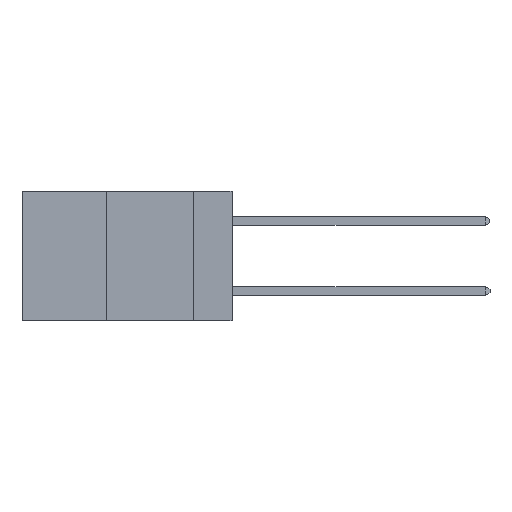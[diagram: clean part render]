
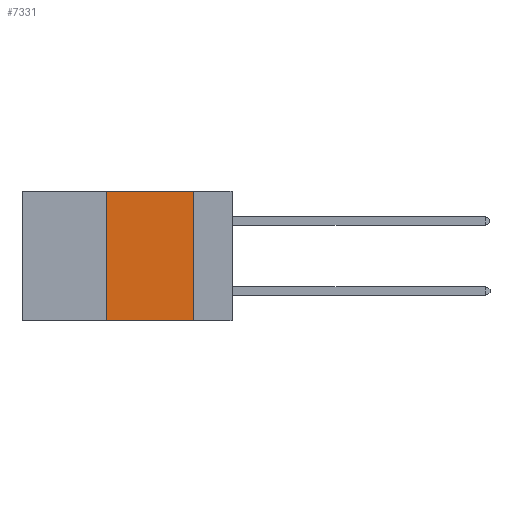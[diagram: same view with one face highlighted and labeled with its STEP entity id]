
A CAD part, left-side view. The second image highlights one B-rep face of the part: STEP entity #7331.
In plain terms, the highlighted planar face has unit normal (-1, 0, 0).
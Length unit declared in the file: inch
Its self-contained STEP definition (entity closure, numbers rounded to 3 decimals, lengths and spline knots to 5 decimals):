
#39 = LINE ( 'NONE', #3463, #8463 ) ;
#714 = ORIENTED_EDGE ( 'NONE', *, *, #12459, .F. ) ;
#884 = DIRECTION ( 'NONE',  ( 0., -1., 0. ) ) ;
#1020 = FACE_OUTER_BOUND ( 'NONE', #5748, .T. ) ;
#1341 = CARTESIAN_POINT ( 'NONE',  ( 0., 0.36, -0.37 ) ) ;
#2169 = VERTEX_POINT ( 'NONE', #8030 ) ;
#2723 = CARTESIAN_POINT ( 'NONE',  ( 0., 0.6, 0. ) ) ;
#2882 = VECTOR ( 'NONE', #884, 39.37008 ) ;
#3002 = EDGE_CURVE ( 'NONE', #5254, #2169, #13405, .T. ) ;
#3463 = CARTESIAN_POINT ( 'NONE',  ( 0., 0.36, 0. ) ) ;
#3580 = CARTESIAN_POINT ( 'NONE',  ( 0., 0.11, 0. ) ) ;
#3927 = VECTOR ( 'NONE', #16142, 39.37008 ) ;
#5190 = EDGE_CURVE ( 'NONE', #8647, #16132, #12346, .T. ) ;
#5254 = VERTEX_POINT ( 'NONE', #1341 ) ;
#5429 = PLANE ( 'NONE',  #18193 ) ;
#5748 = EDGE_LOOP ( 'NONE', ( #714, #13104, #17016, #14029 ) ) ;
#6553 = DIRECTION ( 'NONE',  ( 0., 0., -1. ) ) ;
#7331 = ADVANCED_FACE ( 'NONE', ( #1020 ), #5429, .F. ) ;
#8030 = CARTESIAN_POINT ( 'NONE',  ( 0., 0.11, -0.37 ) ) ;
#8449 = DIRECTION ( 'NONE',  ( 0., 0., -1. ) ) ;
#8463 = VECTOR ( 'NONE', #12419, 39.37008 ) ;
#8647 = VERTEX_POINT ( 'NONE', #14761 ) ;
#9821 = CARTESIAN_POINT ( 'NONE',  ( 0., 0.6, -0.37 ) ) ;
#12346 = LINE ( 'NONE', #2723, #3927 ) ;
#12419 = DIRECTION ( 'NONE',  ( 0., 0., 1. ) ) ;
#12435 = VECTOR ( 'NONE', #6553, 39.37008 ) ;
#12459 = EDGE_CURVE ( 'NONE', #16132, #2169, #17724, .T. ) ;
#13104 = ORIENTED_EDGE ( 'NONE', *, *, #5190, .F. ) ;
#13405 = LINE ( 'NONE', #9821, #2882 ) ;
#14029 = ORIENTED_EDGE ( 'NONE', *, *, #3002, .T. ) ;
#14761 = CARTESIAN_POINT ( 'NONE',  ( 0., 0.36, 0. ) ) ;
#15853 = CARTESIAN_POINT ( 'NONE',  ( 0., 0.6, 0. ) ) ;
#16132 = VERTEX_POINT ( 'NONE', #3580 ) ;
#16142 = DIRECTION ( 'NONE',  ( 0., -1., 0. ) ) ;
#17016 = ORIENTED_EDGE ( 'NONE', *, *, #17441, .F. ) ;
#17330 = DIRECTION ( 'NONE',  ( 1., 0., 0. ) ) ;
#17441 = EDGE_CURVE ( 'NONE', #5254, #8647, #39, .T. ) ;
#17724 = LINE ( 'NONE', #18407, #12435 ) ;
#18193 = AXIS2_PLACEMENT_3D ( 'NONE', #15853, #17330, #8449 ) ;
#18407 = CARTESIAN_POINT ( 'NONE',  ( 0., 0.11, 0. ) ) ;
